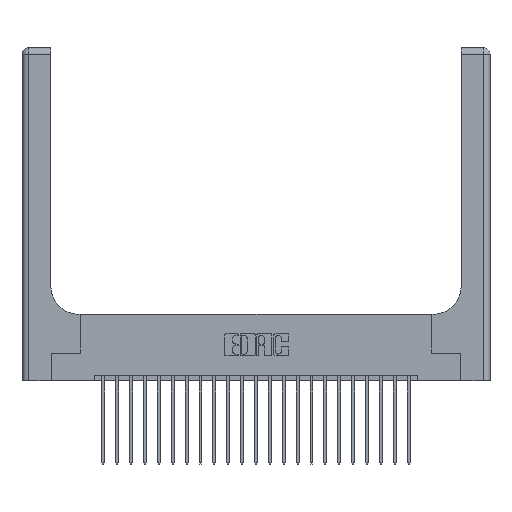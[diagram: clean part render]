
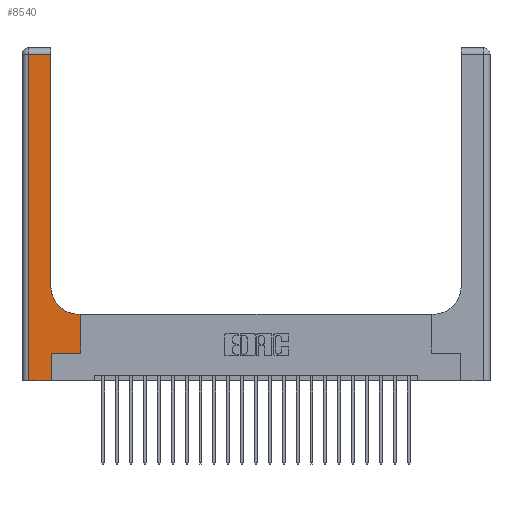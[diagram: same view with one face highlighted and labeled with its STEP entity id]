
A CAD part, top view. The second image highlights one B-rep face of the part: STEP entity #8540.
In plain terms, the highlighted planar face has unit normal (0, 0, 1).
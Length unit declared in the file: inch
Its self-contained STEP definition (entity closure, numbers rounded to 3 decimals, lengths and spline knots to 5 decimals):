
#89 = CARTESIAN_POINT ( 'NONE',  ( 0.265, 0., 0.37 ) ) ;
#469 = CARTESIAN_POINT ( 'NONE',  ( 0.26, 0.85, 0.37 ) ) ;
#609 = DIRECTION ( 'NONE',  ( 0., 1., 0. ) ) ;
#689 = LINE ( 'NONE', #2460, #22768 ) ;
#869 = VECTOR ( 'NONE', #4400, 39.37008 ) ;
#1572 = VERTEX_POINT ( 'NONE', #4652 ) ;
#2254 = EDGE_LOOP ( 'NONE', ( #2774, #9893, #20659, #13788, #23174, #8682, #16813, #10949, #9089 ) ) ;
#2460 = CARTESIAN_POINT ( 'NONE',  ( 0.06, 3., 0.37 ) ) ;
#2690 = LINE ( 'NONE', #4340, #9541 ) ;
#2700 = CARTESIAN_POINT ( 'NONE',  ( 0.51, 0.85, 0.37 ) ) ;
#2774 = ORIENTED_EDGE ( 'NONE', *, *, #6690, .T. ) ;
#4340 = CARTESIAN_POINT ( 'NONE',  ( 0.265, 0.25, 0.37 ) ) ;
#4400 = DIRECTION ( 'NONE',  ( 0., 1., 0. ) ) ;
#4474 = DIRECTION ( 'NONE',  ( 1., 0., 0. ) ) ;
#4578 = DIRECTION ( 'NONE',  ( 1., 0., 0. ) ) ;
#4652 = CARTESIAN_POINT ( 'NONE',  ( 0.528, 0.6, 0.37 ) ) ;
#4931 = VERTEX_POINT ( 'NONE', #8689 ) ;
#5071 = CARTESIAN_POINT ( 'NONE',  ( 0.265, 0., 0.37 ) ) ;
#5118 = VECTOR ( 'NONE', #22773, 39.37008 ) ;
#5713 = EDGE_CURVE ( 'NONE', #13171, #4931, #6079, .T. ) ;
#5881 = DIRECTION ( 'NONE',  ( 0., -1., 0. ) ) ;
#6079 = LINE ( 'NONE', #9573, #20271 ) ;
#6690 = EDGE_CURVE ( 'NONE', #7143, #13171, #8126, .T. ) ;
#7143 = VERTEX_POINT ( 'NONE', #469 ) ;
#8126 = LINE ( 'NONE', #13403, #18399 ) ;
#8448 = CARTESIAN_POINT ( 'NONE',  ( 0.528, 0.25, 0.37 ) ) ;
#8540 = ADVANCED_FACE ( 'NONE', ( #17483 ), #8570, .F. ) ;
#8570 = PLANE ( 'NONE',  #17610 ) ;
#8642 = VERTEX_POINT ( 'NONE', #89 ) ;
#8682 = ORIENTED_EDGE ( 'NONE', *, *, #19231, .T. ) ;
#8689 = CARTESIAN_POINT ( 'NONE',  ( 0.06, 2.94, 0.37 ) ) ;
#8706 = DIRECTION ( 'NONE',  ( 1., 0., 0. ) ) ;
#8812 = VECTOR ( 'NONE', #8706, 39.37008 ) ;
#8838 = EDGE_CURVE ( 'NONE', #1572, #19732, #13821, .T. ) ;
#9089 = ORIENTED_EDGE ( 'NONE', *, *, #9789, .T. ) ;
#9541 = VECTOR ( 'NONE', #4578, 39.37008 ) ;
#9573 = CARTESIAN_POINT ( 'NONE',  ( 0., 2.94, 0.37 ) ) ;
#9789 = EDGE_CURVE ( 'NONE', #19732, #7143, #22906, .T. ) ;
#9893 = ORIENTED_EDGE ( 'NONE', *, *, #5713, .T. ) ;
#10949 = ORIENTED_EDGE ( 'NONE', *, *, #8838, .T. ) ;
#13062 = LINE ( 'NONE', #20247, #8812 ) ;
#13171 = VERTEX_POINT ( 'NONE', #13899 ) ;
#13213 = DIRECTION ( 'NONE',  ( -1., 0., 0. ) ) ;
#13403 = CARTESIAN_POINT ( 'NONE',  ( 0.26, 3., 0.37 ) ) ;
#13437 = EDGE_CURVE ( 'NONE', #22209, #8642, #13062, .T. ) ;
#13788 = ORIENTED_EDGE ( 'NONE', *, *, #13437, .T. ) ;
#13821 = LINE ( 'NONE', #22626, #17995 ) ;
#13899 = CARTESIAN_POINT ( 'NONE',  ( 0.26, 2.94, 0.37 ) ) ;
#13949 = CARTESIAN_POINT ( 'NONE',  ( 0.06, 0., 0.37 ) ) ;
#15060 = EDGE_CURVE ( 'NONE', #8642, #21459, #20471, .T. ) ;
#15320 = CARTESIAN_POINT ( 'NONE',  ( 0.51, 0.6, 0.37 ) ) ;
#15353 = DIRECTION ( 'NONE',  ( -1., 0., 0. ) ) ;
#15737 = DIRECTION ( 'NONE',  ( 0., 0., -1. ) ) ;
#16160 = AXIS2_PLACEMENT_3D ( 'NONE', #2700, #22194, #4474 ) ;
#16813 = ORIENTED_EDGE ( 'NONE', *, *, #20396, .T. ) ;
#17483 = FACE_OUTER_BOUND ( 'NONE', #2254, .T. ) ;
#17610 = AXIS2_PLACEMENT_3D ( 'NONE', #17615, #15737, #18891 ) ;
#17615 = CARTESIAN_POINT ( 'NONE',  ( 0., 3., 0.37 ) ) ;
#17995 = VECTOR ( 'NONE', #15353, 39.37008 ) ;
#18096 = VERTEX_POINT ( 'NONE', #21994 ) ;
#18399 = VECTOR ( 'NONE', #609, 39.37008 ) ;
#18891 = DIRECTION ( 'NONE',  ( -1., 0., 0. ) ) ;
#19129 = LINE ( 'NONE', #8448, #5118 ) ;
#19231 = EDGE_CURVE ( 'NONE', #21459, #18096, #2690, .T. ) ;
#19732 = VERTEX_POINT ( 'NONE', #15320 ) ;
#19874 = CARTESIAN_POINT ( 'NONE',  ( 0.265, 0.25, 0.37 ) ) ;
#20247 = CARTESIAN_POINT ( 'NONE',  ( 0., 0., 0.37 ) ) ;
#20271 = VECTOR ( 'NONE', #13213, 39.37008 ) ;
#20396 = EDGE_CURVE ( 'NONE', #18096, #1572, #19129, .T. ) ;
#20471 = LINE ( 'NONE', #5071, #869 ) ;
#20659 = ORIENTED_EDGE ( 'NONE', *, *, #21903, .T. ) ;
#21459 = VERTEX_POINT ( 'NONE', #19874 ) ;
#21903 = EDGE_CURVE ( 'NONE', #4931, #22209, #689, .T. ) ;
#21994 = CARTESIAN_POINT ( 'NONE',  ( 0.528, 0.25, 0.37 ) ) ;
#22194 = DIRECTION ( 'NONE',  ( 0., 0., -1. ) ) ;
#22209 = VERTEX_POINT ( 'NONE', #13949 ) ;
#22626 = CARTESIAN_POINT ( 'NONE',  ( 0.26, 0.6, 0.37 ) ) ;
#22768 = VECTOR ( 'NONE', #5881, 39.37008 ) ;
#22773 = DIRECTION ( 'NONE',  ( 0., 1., 0. ) ) ;
#22906 = CIRCLE ( 'NONE', #16160, 0.25 ) ;
#23174 = ORIENTED_EDGE ( 'NONE', *, *, #15060, .T. ) ;
